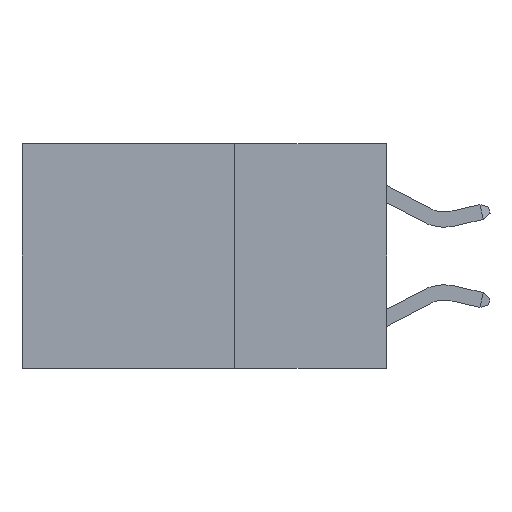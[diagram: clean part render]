
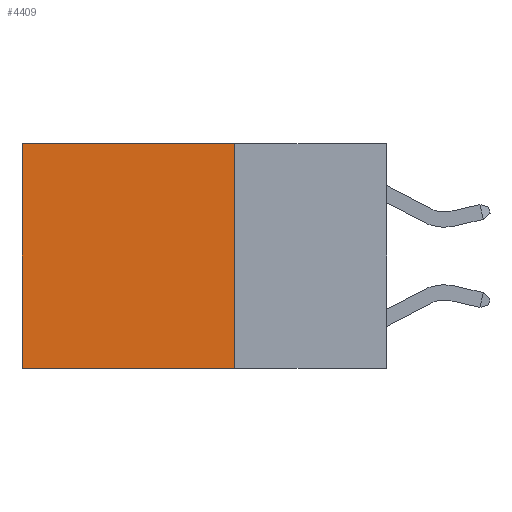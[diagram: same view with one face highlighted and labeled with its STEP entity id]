
A CAD part, left-side view. The second image highlights one B-rep face of the part: STEP entity #4409.
In plain terms, the highlighted planar face has unit normal (-1, 0, 0).
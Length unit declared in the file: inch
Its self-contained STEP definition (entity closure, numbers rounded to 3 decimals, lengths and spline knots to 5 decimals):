
#340 = LINE ( 'NONE', #13344, #17666 ) ;
#1252 = ORIENTED_EDGE ( 'NONE', *, *, #2441, .T. ) ;
#1797 = ORIENTED_EDGE ( 'NONE', *, *, #14969, .T. ) ;
#2256 = LINE ( 'NONE', #14402, #2500 ) ;
#2441 = EDGE_CURVE ( 'NONE', #20391, #12667, #340, .T. ) ;
#2462 = CARTESIAN_POINT ( 'NONE',  ( 0.2625, 0.6, 0. ) ) ;
#2500 = VECTOR ( 'NONE', #12892, 39.37008 ) ;
#4409 = ADVANCED_FACE ( 'NONE', ( #9047 ), #18053, .F. ) ;
#4499 = CARTESIAN_POINT ( 'NONE',  ( 0.2625, 0.6, -0.37 ) ) ;
#5951 = VECTOR ( 'NONE', #8918, 39.37008 ) ;
#6696 = EDGE_CURVE ( 'NONE', #19596, #12667, #2256, .T. ) ;
#7731 = ORIENTED_EDGE ( 'NONE', *, *, #20944, .F. ) ;
#7843 = AXIS2_PLACEMENT_3D ( 'NONE', #8152, #8359, #16559 ) ;
#8152 = CARTESIAN_POINT ( 'NONE',  ( 0.2625, 0.25, 0. ) ) ;
#8359 = DIRECTION ( 'NONE',  ( 1., 0., 0. ) ) ;
#8639 = CARTESIAN_POINT ( 'NONE',  ( 0.2625, 0.25, 0. ) ) ;
#8836 = DIRECTION ( 'NONE',  ( 0., 0., -1. ) ) ;
#8918 = DIRECTION ( 'NONE',  ( 0., 1., 0. ) ) ;
#9047 = FACE_OUTER_BOUND ( 'NONE', #16155, .T. ) ;
#11259 = VERTEX_POINT ( 'NONE', #8639 ) ;
#12667 = VERTEX_POINT ( 'NONE', #4499 ) ;
#12892 = DIRECTION ( 'NONE',  ( 0., 1., 0. ) ) ;
#13344 = CARTESIAN_POINT ( 'NONE',  ( 0.2625, 0.6, 0. ) ) ;
#13413 = CARTESIAN_POINT ( 'NONE',  ( 0.2625, 0.25, 0. ) ) ;
#14402 = CARTESIAN_POINT ( 'NONE',  ( 0.2625, 0.25, -0.37 ) ) ;
#14491 = LINE ( 'NONE', #15499, #5951 ) ;
#14901 = CARTESIAN_POINT ( 'NONE',  ( 0.2625, 0.25, -0.37 ) ) ;
#14969 = EDGE_CURVE ( 'NONE', #11259, #20391, #14491, .T. ) ;
#15499 = CARTESIAN_POINT ( 'NONE',  ( 0.2625, 0.25, 0. ) ) ;
#16078 = ORIENTED_EDGE ( 'NONE', *, *, #6696, .F. ) ;
#16155 = EDGE_LOOP ( 'NONE', ( #1252, #16078, #7731, #1797 ) ) ;
#16559 = DIRECTION ( 'NONE',  ( 0., 0., -1. ) ) ;
#17666 = VECTOR ( 'NONE', #20111, 39.37008 ) ;
#18053 = PLANE ( 'NONE',  #7843 ) ;
#19596 = VERTEX_POINT ( 'NONE', #14901 ) ;
#20032 = LINE ( 'NONE', #13413, #20501 ) ;
#20111 = DIRECTION ( 'NONE',  ( 0., 0., -1. ) ) ;
#20391 = VERTEX_POINT ( 'NONE', #2462 ) ;
#20501 = VECTOR ( 'NONE', #8836, 39.37008 ) ;
#20944 = EDGE_CURVE ( 'NONE', #11259, #19596, #20032, .T. ) ;
